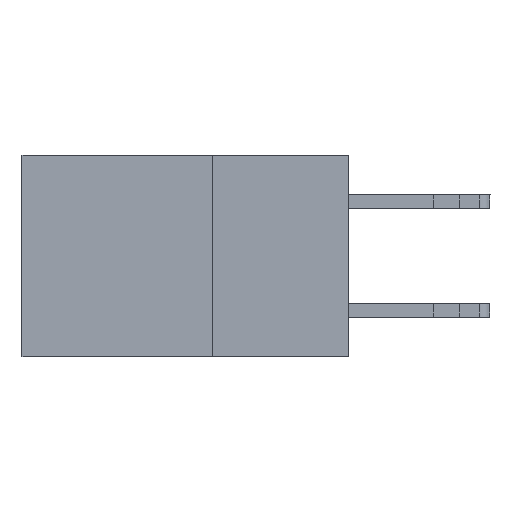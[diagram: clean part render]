
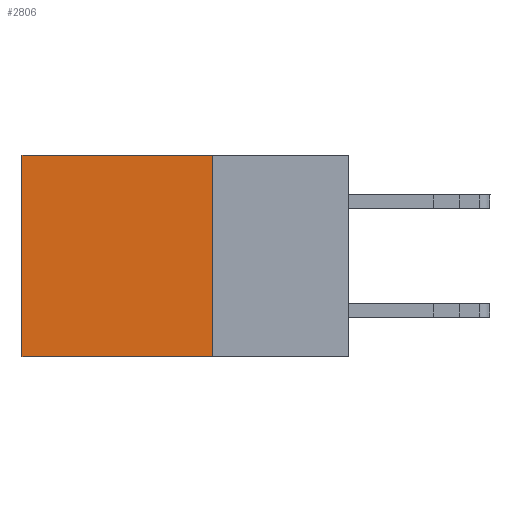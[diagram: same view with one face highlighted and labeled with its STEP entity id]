
A CAD part, left-side view. The second image highlights one B-rep face of the part: STEP entity #2806.
In plain terms, the highlighted planar face has unit normal (-1, 0, 0).
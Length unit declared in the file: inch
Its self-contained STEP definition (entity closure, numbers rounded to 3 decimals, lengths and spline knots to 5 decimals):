
#506 = DIRECTION ( 'NONE',  ( 0., 0., -1. ) ) ;
#904 = CARTESIAN_POINT ( 'NONE',  ( 0.298, 0.6, 0. ) ) ;
#2081 = CARTESIAN_POINT ( 'NONE',  ( 0.298, 0.6, 0. ) ) ;
#2468 = CARTESIAN_POINT ( 'NONE',  ( 0.298, 0.6, -0.37 ) ) ;
#2806 = ADVANCED_FACE ( 'NONE', ( #19787 ), #9292, .F. ) ;
#2878 = ORIENTED_EDGE ( 'NONE', *, *, #14808, .F. ) ;
#3407 = CARTESIAN_POINT ( 'NONE',  ( 0.298, 0.25, 0. ) ) ;
#5880 = CARTESIAN_POINT ( 'NONE',  ( 0.298, 0.25, 0. ) ) ;
#6194 = DIRECTION ( 'NONE',  ( 0., 1., 0. ) ) ;
#7382 = DIRECTION ( 'NONE',  ( 0., 0., -1. ) ) ;
#7442 = AXIS2_PLACEMENT_3D ( 'NONE', #5880, #16559, #16108 ) ;
#7500 = DIRECTION ( 'NONE',  ( 0., 1., 0. ) ) ;
#8647 = EDGE_CURVE ( 'NONE', #18640, #10935, #14843, .T. ) ;
#9292 = PLANE ( 'NONE',  #7442 ) ;
#9710 = VERTEX_POINT ( 'NONE', #19881 ) ;
#10445 = ORIENTED_EDGE ( 'NONE', *, *, #18794, .T. ) ;
#10587 = LINE ( 'NONE', #2081, #19575 ) ;
#10674 = EDGE_LOOP ( 'NONE', ( #10445, #2878, #19413, #17157 ) ) ;
#10935 = VERTEX_POINT ( 'NONE', #904 ) ;
#11274 = CARTESIAN_POINT ( 'NONE',  ( 0.298, 0.25, 0. ) ) ;
#11704 = VECTOR ( 'NONE', #6194, 39.37008 ) ;
#12128 = EDGE_CURVE ( 'NONE', #18640, #9710, #17024, .T. ) ;
#12340 = CARTESIAN_POINT ( 'NONE',  ( 0.298, 0.25, 0. ) ) ;
#14808 = EDGE_CURVE ( 'NONE', #9710, #21179, #20708, .T. ) ;
#14843 = LINE ( 'NONE', #11274, #11704 ) ;
#15686 = CARTESIAN_POINT ( 'NONE',  ( 0.298, 0.25, -0.37 ) ) ;
#16108 = DIRECTION ( 'NONE',  ( 0., 0., -1. ) ) ;
#16559 = DIRECTION ( 'NONE',  ( 1., 0., 0. ) ) ;
#17024 = LINE ( 'NONE', #12340, #20077 ) ;
#17157 = ORIENTED_EDGE ( 'NONE', *, *, #8647, .T. ) ;
#17907 = VECTOR ( 'NONE', #7500, 39.37008 ) ;
#18640 = VERTEX_POINT ( 'NONE', #3407 ) ;
#18794 = EDGE_CURVE ( 'NONE', #10935, #21179, #10587, .T. ) ;
#19413 = ORIENTED_EDGE ( 'NONE', *, *, #12128, .F. ) ;
#19575 = VECTOR ( 'NONE', #506, 39.37008 ) ;
#19787 = FACE_OUTER_BOUND ( 'NONE', #10674, .T. ) ;
#19881 = CARTESIAN_POINT ( 'NONE',  ( 0.298, 0.25, -0.37 ) ) ;
#20077 = VECTOR ( 'NONE', #7382, 39.37008 ) ;
#20708 = LINE ( 'NONE', #15686, #17907 ) ;
#21179 = VERTEX_POINT ( 'NONE', #2468 ) ;
